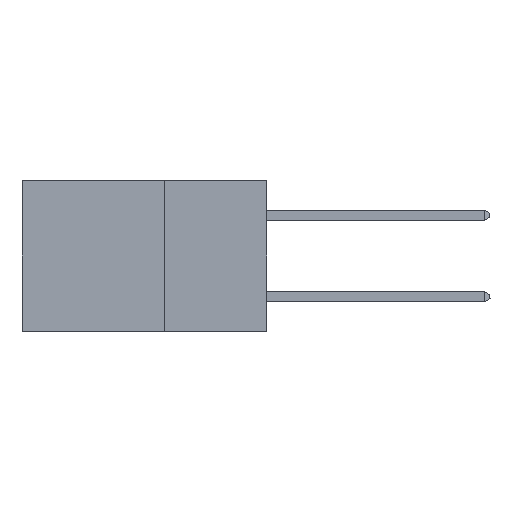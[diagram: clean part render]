
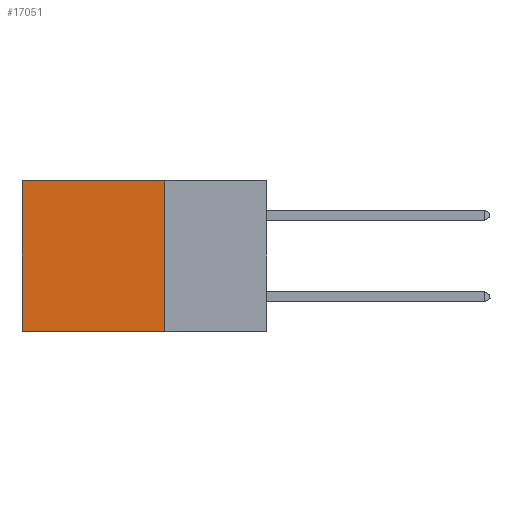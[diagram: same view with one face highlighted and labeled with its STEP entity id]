
A CAD part, left-side view. The second image highlights one B-rep face of the part: STEP entity #17051.
In plain terms, the highlighted planar face has unit normal (-1, 0, 0).
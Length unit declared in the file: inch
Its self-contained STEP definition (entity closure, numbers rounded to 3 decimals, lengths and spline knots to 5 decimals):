
#3058 = CARTESIAN_POINT ( 'NONE',  ( 0.2875, 0.25, -0.37 ) ) ;
#4331 = LINE ( 'NONE', #14654, #9072 ) ;
#4600 = EDGE_CURVE ( 'NONE', #23595, #17944, #4331, .T. ) ;
#4603 = FACE_OUTER_BOUND ( 'NONE', #6717, .T. ) ;
#4802 = VERTEX_POINT ( 'NONE', #13050 ) ;
#5468 = LINE ( 'NONE', #20767, #23097 ) ;
#6717 = EDGE_LOOP ( 'NONE', ( #27182, #7216, #16943, #23900 ) ) ;
#6790 = CARTESIAN_POINT ( 'NONE',  ( 0.2875, 0.25, -0.37 ) ) ;
#7216 = ORIENTED_EDGE ( 'NONE', *, *, #16918, .F. ) ;
#7493 = LINE ( 'NONE', #3058, #25092 ) ;
#8131 = EDGE_CURVE ( 'NONE', #23595, #16664, #5468, .T. ) ;
#9072 = VECTOR ( 'NONE', #16949, 39.37008 ) ;
#9431 = AXIS2_PLACEMENT_3D ( 'NONE', #19572, #10530, #26432 ) ;
#9724 = EDGE_CURVE ( 'NONE', #16664, #4802, #23737, .T. ) ;
#10530 = DIRECTION ( 'NONE',  ( 1., 0., 0. ) ) ;
#12099 = CARTESIAN_POINT ( 'NONE',  ( 0.2875, 0.25, 0. ) ) ;
#13050 = CARTESIAN_POINT ( 'NONE',  ( 0.2875, 0.6, -0.37 ) ) ;
#14654 = CARTESIAN_POINT ( 'NONE',  ( 0.2875, 0.25, 0. ) ) ;
#15079 = PLANE ( 'NONE',  #9431 ) ;
#16664 = VERTEX_POINT ( 'NONE', #17758 ) ;
#16918 = EDGE_CURVE ( 'NONE', #17944, #4802, #7493, .T. ) ;
#16943 = ORIENTED_EDGE ( 'NONE', *, *, #4600, .F. ) ;
#16949 = DIRECTION ( 'NONE',  ( 0., 0., -1. ) ) ;
#17051 = ADVANCED_FACE ( 'NONE', ( #4603 ), #15079, .F. ) ;
#17758 = CARTESIAN_POINT ( 'NONE',  ( 0.2875, 0.6, 0. ) ) ;
#17759 = VECTOR ( 'NONE', #28120, 39.37008 ) ;
#17944 = VERTEX_POINT ( 'NONE', #6790 ) ;
#19572 = CARTESIAN_POINT ( 'NONE',  ( 0.2875, 0.25, 0. ) ) ;
#20767 = CARTESIAN_POINT ( 'NONE',  ( 0.2875, 0.25, 0. ) ) ;
#21517 = DIRECTION ( 'NONE',  ( 0., 1., 0. ) ) ;
#23097 = VECTOR ( 'NONE', #25206, 39.37008 ) ;
#23595 = VERTEX_POINT ( 'NONE', #12099 ) ;
#23737 = LINE ( 'NONE', #25695, #17759 ) ;
#23900 = ORIENTED_EDGE ( 'NONE', *, *, #8131, .T. ) ;
#25092 = VECTOR ( 'NONE', #21517, 39.37008 ) ;
#25206 = DIRECTION ( 'NONE',  ( 0., 1., 0. ) ) ;
#25695 = CARTESIAN_POINT ( 'NONE',  ( 0.2875, 0.6, 0. ) ) ;
#26432 = DIRECTION ( 'NONE',  ( 0., 0., -1. ) ) ;
#27182 = ORIENTED_EDGE ( 'NONE', *, *, #9724, .T. ) ;
#28120 = DIRECTION ( 'NONE',  ( 0., 0., -1. ) ) ;
